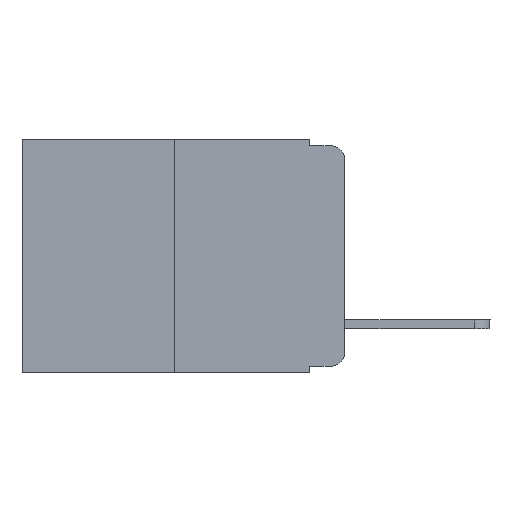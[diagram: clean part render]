
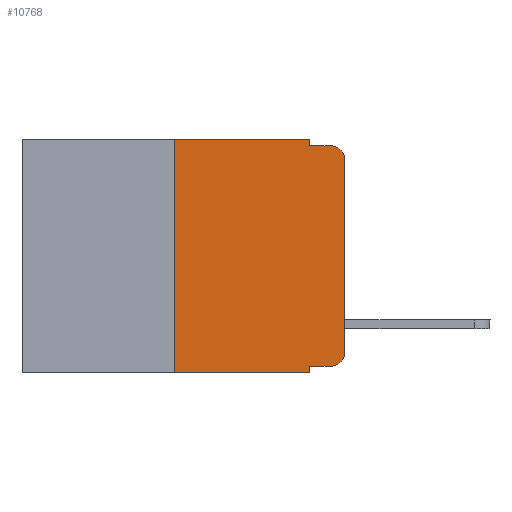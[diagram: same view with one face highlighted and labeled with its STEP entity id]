
A CAD part, left-side view. The second image highlights one B-rep face of the part: STEP entity #10768.
In plain terms, the highlighted planar face has unit normal (-1, 0, 0).
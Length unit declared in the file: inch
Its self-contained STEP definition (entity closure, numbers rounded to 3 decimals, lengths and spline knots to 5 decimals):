
#52 = VECTOR ( 'NONE', #3563, 39.37008 ) ;
#324 = VECTOR ( 'NONE', #9847, 39.37008 ) ;
#698 = AXIS2_PLACEMENT_3D ( 'NONE', #16836, #10800, #1894 ) ;
#787 = CARTESIAN_POINT ( 'NONE',  ( 0., 0.02, -0.333 ) ) ;
#788 = CARTESIAN_POINT ( 'NONE',  ( 0., 0.051, -0.333 ) ) ;
#965 = DIRECTION ( 'NONE',  ( 0., -1., 0. ) ) ;
#1229 = DIRECTION ( 'NONE',  ( 0., 0., -1. ) ) ;
#1393 = VERTEX_POINT ( 'NONE', #18882 ) ;
#1894 = DIRECTION ( 'NONE',  ( 0., 0., -1. ) ) ;
#2748 = DIRECTION ( 'NONE',  ( 0., -1., 0. ) ) ;
#2845 = DIRECTION ( 'NONE',  ( -1., 0., 0. ) ) ;
#3122 = FACE_OUTER_BOUND ( 'NONE', #18558, .T. ) ;
#3187 = CARTESIAN_POINT ( 'NONE',  ( 0., 0.473, 0. ) ) ;
#3200 = ORIENTED_EDGE ( 'NONE', *, *, #3776, .T. ) ;
#3209 = LINE ( 'NONE', #16258, #7710 ) ;
#3563 = DIRECTION ( 'NONE',  ( 0., -1., 0. ) ) ;
#3583 = AXIS2_PLACEMENT_3D ( 'NONE', #3187, #10659, #8926 ) ;
#3776 = EDGE_CURVE ( 'NONE', #1393, #6225, #6631, .T. ) ;
#3801 = VECTOR ( 'NONE', #1229, 39.37008 ) ;
#4058 = ORIENTED_EDGE ( 'NONE', *, *, #14660, .T. ) ;
#4066 = EDGE_CURVE ( 'NONE', #10670, #7436, #13933, .T. ) ;
#4104 = CARTESIAN_POINT ( 'NONE',  ( 0., 0.051, -0.343 ) ) ;
#4122 = CARTESIAN_POINT ( 'NONE',  ( 0., 0.051, -0.01 ) ) ;
#4527 = CARTESIAN_POINT ( 'NONE',  ( 0., 0.473, 0. ) ) ;
#4879 = VERTEX_POINT ( 'NONE', #6943 ) ;
#4963 = CARTESIAN_POINT ( 'NONE',  ( 0., 0.02, -0.01 ) ) ;
#4977 = LINE ( 'NONE', #10709, #9670 ) ;
#5058 = ORIENTED_EDGE ( 'NONE', *, *, #10537, .T. ) ;
#5452 = CARTESIAN_POINT ( 'NONE',  ( 0., 0.25, 0. ) ) ;
#5472 = CARTESIAN_POINT ( 'NONE',  ( 0., 0.25, -0.343 ) ) ;
#5554 = EDGE_CURVE ( 'NONE', #17721, #4879, #13990, .T. ) ;
#5857 = LINE ( 'NONE', #4527, #17876 ) ;
#5986 = PLANE ( 'NONE',  #3583 ) ;
#6077 = DIRECTION ( 'NONE',  ( 0., 0., -1. ) ) ;
#6175 = LINE ( 'NONE', #16363, #3801 ) ;
#6225 = VERTEX_POINT ( 'NONE', #787 ) ;
#6557 = EDGE_CURVE ( 'NONE', #4879, #11648, #5857, .T. ) ;
#6631 = LINE ( 'NONE', #788, #52 ) ;
#6737 = ORIENTED_EDGE ( 'NONE', *, *, #11897, .T. ) ;
#6943 = CARTESIAN_POINT ( 'NONE',  ( 0., 0.25, 0. ) ) ;
#6948 = CIRCLE ( 'NONE', #18396, 0.02 ) ;
#7256 = CARTESIAN_POINT ( 'NONE',  ( 0., 0.051, 0. ) ) ;
#7436 = VERTEX_POINT ( 'NONE', #4963 ) ;
#7570 = VERTEX_POINT ( 'NONE', #14297 ) ;
#7710 = VECTOR ( 'NONE', #14556, 39.37008 ) ;
#8696 = VERTEX_POINT ( 'NONE', #4104 ) ;
#8926 = DIRECTION ( 'NONE',  ( 0., 0., -1. ) ) ;
#9338 = VERTEX_POINT ( 'NONE', #13475 ) ;
#9670 = VECTOR ( 'NONE', #16756, 39.37008 ) ;
#9847 = DIRECTION ( 'NONE',  ( 0., 0., 1. ) ) ;
#9851 = CARTESIAN_POINT ( 'NONE',  ( 0., 0.473, -0.343 ) ) ;
#10537 = EDGE_CURVE ( 'NONE', #17721, #8696, #14672, .T. ) ;
#10659 = DIRECTION ( 'NONE',  ( 1., 0., 0. ) ) ;
#10670 = VERTEX_POINT ( 'NONE', #16369 ) ;
#10709 = CARTESIAN_POINT ( 'NONE',  ( 0., 0., 0. ) ) ;
#10768 = ADVANCED_FACE ( 'NONE', ( #3122 ), #5986, .F. ) ;
#10800 = DIRECTION ( 'NONE',  ( -1., 0., 0. ) ) ;
#10907 = VECTOR ( 'NONE', #965, 39.37008 ) ;
#11295 = ORIENTED_EDGE ( 'NONE', *, *, #19432, .T. ) ;
#11648 = VERTEX_POINT ( 'NONE', #7256 ) ;
#11897 = EDGE_CURVE ( 'NONE', #9338, #7436, #15437, .T. ) ;
#12083 = ORIENTED_EDGE ( 'NONE', *, *, #4066, .F. ) ;
#12093 = ORIENTED_EDGE ( 'NONE', *, *, #19273, .F. ) ;
#13475 = CARTESIAN_POINT ( 'NONE',  ( 0., 0., -0.03 ) ) ;
#13933 = LINE ( 'NONE', #4122, #19344 ) ;
#13990 = LINE ( 'NONE', #5452, #324 ) ;
#14297 = CARTESIAN_POINT ( 'NONE',  ( 0., 0., -0.313 ) ) ;
#14556 = DIRECTION ( 'NONE',  ( 0., 0., -1. ) ) ;
#14660 = EDGE_CURVE ( 'NONE', #6225, #7570, #6948, .T. ) ;
#14672 = LINE ( 'NONE', #9851, #10907 ) ;
#15351 = ORIENTED_EDGE ( 'NONE', *, *, #6557, .F. ) ;
#15437 = CIRCLE ( 'NONE', #698, 0.02 ) ;
#15740 = ORIENTED_EDGE ( 'NONE', *, *, #17692, .F. ) ;
#16258 = CARTESIAN_POINT ( 'NONE',  ( 0., 0.051, 0. ) ) ;
#16363 = CARTESIAN_POINT ( 'NONE',  ( 0., 0.051, 0. ) ) ;
#16369 = CARTESIAN_POINT ( 'NONE',  ( 0., 0.051, -0.01 ) ) ;
#16756 = DIRECTION ( 'NONE',  ( 0., 0., 1. ) ) ;
#16836 = CARTESIAN_POINT ( 'NONE',  ( 0., 0.02, -0.03 ) ) ;
#17692 = EDGE_CURVE ( 'NONE', #1393, #8696, #3209, .T. ) ;
#17721 = VERTEX_POINT ( 'NONE', #5472 ) ;
#17747 = ORIENTED_EDGE ( 'NONE', *, *, #5554, .F. ) ;
#17876 = VECTOR ( 'NONE', #17904, 39.37008 ) ;
#17904 = DIRECTION ( 'NONE',  ( 0., -1., 0. ) ) ;
#18063 = CARTESIAN_POINT ( 'NONE',  ( 0., 0.02, -0.313 ) ) ;
#18396 = AXIS2_PLACEMENT_3D ( 'NONE', #18063, #2845, #6077 ) ;
#18558 = EDGE_LOOP ( 'NONE', ( #11295, #6737, #12083, #12093, #15351, #17747, #5058, #15740, #3200, #4058 ) ) ;
#18882 = CARTESIAN_POINT ( 'NONE',  ( 0., 0.051, -0.333 ) ) ;
#19273 = EDGE_CURVE ( 'NONE', #11648, #10670, #6175, .T. ) ;
#19344 = VECTOR ( 'NONE', #2748, 39.37008 ) ;
#19432 = EDGE_CURVE ( 'NONE', #7570, #9338, #4977, .T. ) ;
